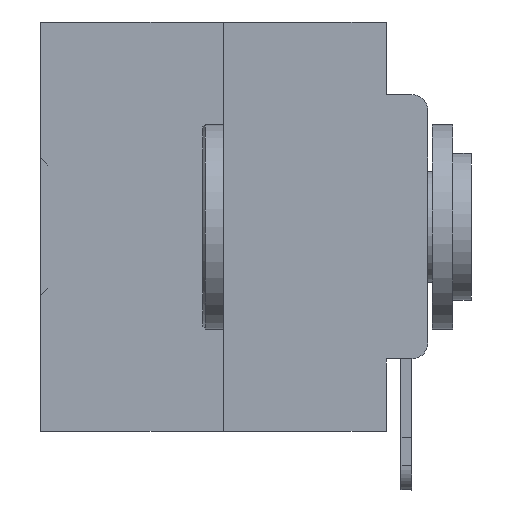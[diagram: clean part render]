
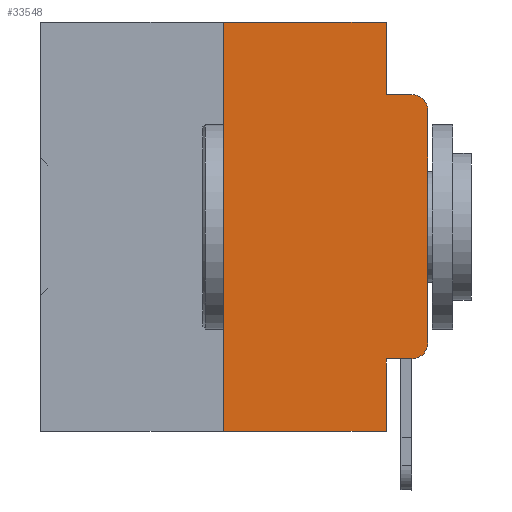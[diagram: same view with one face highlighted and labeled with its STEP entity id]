
A CAD part, left-side view. The second image highlights one B-rep face of the part: STEP entity #33548.
In plain terms, the highlighted planar face has unit normal (-1, 0, 0).
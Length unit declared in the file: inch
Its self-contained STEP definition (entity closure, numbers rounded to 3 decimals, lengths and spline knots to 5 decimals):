
#548 = CARTESIAN_POINT ( 'NONE',  ( 0., 0.051, -0.5 ) ) ;
#608 = VERTEX_POINT ( 'NONE', #32886 ) ;
#837 = ORIENTED_EDGE ( 'NONE', *, *, #10808, .F. ) ;
#919 = DIRECTION ( 'NONE',  ( -1., 0., 0. ) ) ;
#1111 = DIRECTION ( 'NONE',  ( 0., 0., -1. ) ) ;
#1181 = CARTESIAN_POINT ( 'NONE',  ( 0., 0., 0. ) ) ;
#1508 = VERTEX_POINT ( 'NONE', #24649 ) ;
#1780 = ORIENTED_EDGE ( 'NONE', *, *, #22128, .F. ) ;
#2645 = EDGE_CURVE ( 'NONE', #16327, #608, #9217, .T. ) ;
#2679 = EDGE_CURVE ( 'NONE', #608, #12164, #24099, .T. ) ;
#2886 = DIRECTION ( 'NONE',  ( 0., -1., 0. ) ) ;
#3050 = FACE_OUTER_BOUND ( 'NONE', #23467, .T. ) ;
#3422 = DIRECTION ( 'NONE',  ( 1., 0., 0. ) ) ;
#3719 = VERTEX_POINT ( 'NONE', #8163 ) ;
#4757 = LINE ( 'NONE', #15724, #26916 ) ;
#4942 = VECTOR ( 'NONE', #21710, 39.37008 ) ;
#6395 = CARTESIAN_POINT ( 'NONE',  ( 0., 0., -0.1085 ) ) ;
#6479 = AXIS2_PLACEMENT_3D ( 'NONE', #17713, #28826, #26559 ) ;
#7093 = CARTESIAN_POINT ( 'NONE',  ( 0., 0.051, -0.4115 ) ) ;
#7149 = DIRECTION ( 'NONE',  ( 0., 0., -1. ) ) ;
#7471 = AXIS2_PLACEMENT_3D ( 'NONE', #18282, #919, #7149 ) ;
#8163 = CARTESIAN_POINT ( 'NONE',  ( 0., 0.25, -0.5 ) ) ;
#9049 = VECTOR ( 'NONE', #33107, 39.37008 ) ;
#9217 = LINE ( 'NONE', #32236, #19100 ) ;
#9265 = CIRCLE ( 'NONE', #7471, 0.02 ) ;
#9586 = CARTESIAN_POINT ( 'NONE',  ( 0., 0.02, -0.4115 ) ) ;
#9649 = LINE ( 'NONE', #1181, #31428 ) ;
#10416 = VECTOR ( 'NONE', #30965, 39.37008 ) ;
#10808 = EDGE_CURVE ( 'NONE', #12164, #1508, #23047, .T. ) ;
#12164 = VERTEX_POINT ( 'NONE', #26993 ) ;
#12439 = VERTEX_POINT ( 'NONE', #9586 ) ;
#12482 = VERTEX_POINT ( 'NONE', #548 ) ;
#12674 = DIRECTION ( 'NONE',  ( 0., 0., 1. ) ) ;
#13782 = ORIENTED_EDGE ( 'NONE', *, *, #24115, .T. ) ;
#14307 = CIRCLE ( 'NONE', #6479, 0.02 ) ;
#14481 = CARTESIAN_POINT ( 'NONE',  ( 0., 0.25, 0. ) ) ;
#15062 = DIRECTION ( 'NONE',  ( 0., -1., 0. ) ) ;
#15133 = DIRECTION ( 'NONE',  ( 0., 0., 1. ) ) ;
#15469 = EDGE_CURVE ( 'NONE', #18313, #24036, #9649, .T. ) ;
#15624 = ORIENTED_EDGE ( 'NONE', *, *, #27233, .T. ) ;
#15724 = CARTESIAN_POINT ( 'NONE',  ( 0., 0.25, 0. ) ) ;
#15739 = CARTESIAN_POINT ( 'NONE',  ( 0., 0., -0.3915 ) ) ;
#16259 = LINE ( 'NONE', #30570, #4942 ) ;
#16327 = VERTEX_POINT ( 'NONE', #14481 ) ;
#17713 = CARTESIAN_POINT ( 'NONE',  ( 0., 0.02, -0.3915 ) ) ;
#18282 = CARTESIAN_POINT ( 'NONE',  ( 0., 0.02, -0.1085 ) ) ;
#18313 = VERTEX_POINT ( 'NONE', #15739 ) ;
#19100 = VECTOR ( 'NONE', #15062, 39.37008 ) ;
#19272 = ORIENTED_EDGE ( 'NONE', *, *, #36979, .F. ) ;
#19282 = LINE ( 'NONE', #30590, #10416 ) ;
#21408 = LINE ( 'NONE', #7093, #9049 ) ;
#21710 = DIRECTION ( 'NONE',  ( 0., 0., -1. ) ) ;
#22128 = EDGE_CURVE ( 'NONE', #3719, #16327, #4757, .T. ) ;
#22302 = CARTESIAN_POINT ( 'NONE',  ( 0., 0.051, -0.0885 ) ) ;
#23047 = LINE ( 'NONE', #22302, #36288 ) ;
#23467 = EDGE_LOOP ( 'NONE', ( #29989, #24654, #837, #31846, #28442, #1780, #26478, #19272, #15624, #13782 ) ) ;
#23967 = CARTESIAN_POINT ( 'NONE',  ( 0., 0.051, -0.4115 ) ) ;
#24036 = VERTEX_POINT ( 'NONE', #6395 ) ;
#24099 = LINE ( 'NONE', #33356, #35991 ) ;
#24115 = EDGE_CURVE ( 'NONE', #12439, #18313, #14307, .T. ) ;
#24649 = CARTESIAN_POINT ( 'NONE',  ( 0., 0.02, -0.0885 ) ) ;
#24654 = ORIENTED_EDGE ( 'NONE', *, *, #32021, .T. ) ;
#26240 = PLANE ( 'NONE',  #26812 ) ;
#26478 = ORIENTED_EDGE ( 'NONE', *, *, #31284, .T. ) ;
#26559 = DIRECTION ( 'NONE',  ( 0., 0., -1. ) ) ;
#26812 = AXIS2_PLACEMENT_3D ( 'NONE', #29254, #3422, #29436 ) ;
#26916 = VECTOR ( 'NONE', #12674, 39.37008 ) ;
#26993 = CARTESIAN_POINT ( 'NONE',  ( 0., 0.051, -0.0885 ) ) ;
#27233 = EDGE_CURVE ( 'NONE', #31553, #12439, #21408, .T. ) ;
#28442 = ORIENTED_EDGE ( 'NONE', *, *, #2645, .F. ) ;
#28826 = DIRECTION ( 'NONE',  ( -1., 0., 0. ) ) ;
#29254 = CARTESIAN_POINT ( 'NONE',  ( 0., 0.473, 0. ) ) ;
#29436 = DIRECTION ( 'NONE',  ( 0., 0., -1. ) ) ;
#29989 = ORIENTED_EDGE ( 'NONE', *, *, #15469, .T. ) ;
#30570 = CARTESIAN_POINT ( 'NONE',  ( 0., 0.051, 0. ) ) ;
#30590 = CARTESIAN_POINT ( 'NONE',  ( 0., 0.473, -0.5 ) ) ;
#30965 = DIRECTION ( 'NONE',  ( 0., -1., 0. ) ) ;
#31284 = EDGE_CURVE ( 'NONE', #3719, #12482, #19282, .T. ) ;
#31428 = VECTOR ( 'NONE', #15133, 39.37008 ) ;
#31553 = VERTEX_POINT ( 'NONE', #23967 ) ;
#31846 = ORIENTED_EDGE ( 'NONE', *, *, #2679, .F. ) ;
#32021 = EDGE_CURVE ( 'NONE', #24036, #1508, #9265, .T. ) ;
#32236 = CARTESIAN_POINT ( 'NONE',  ( 0., 0.473, 0. ) ) ;
#32886 = CARTESIAN_POINT ( 'NONE',  ( 0., 0.051, 0. ) ) ;
#33107 = DIRECTION ( 'NONE',  ( 0., -1., 0. ) ) ;
#33356 = CARTESIAN_POINT ( 'NONE',  ( 0., 0.051, 0. ) ) ;
#33548 = ADVANCED_FACE ( 'NONE', ( #3050 ), #26240, .F. ) ;
#35991 = VECTOR ( 'NONE', #1111, 39.37008 ) ;
#36288 = VECTOR ( 'NONE', #2886, 39.37008 ) ;
#36979 = EDGE_CURVE ( 'NONE', #31553, #12482, #16259, .T. ) ;
